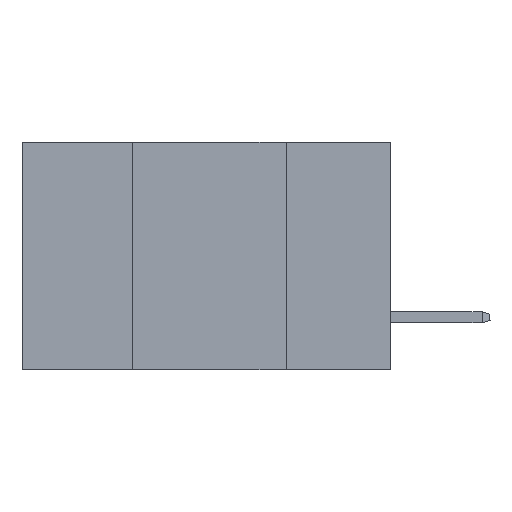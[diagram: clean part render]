
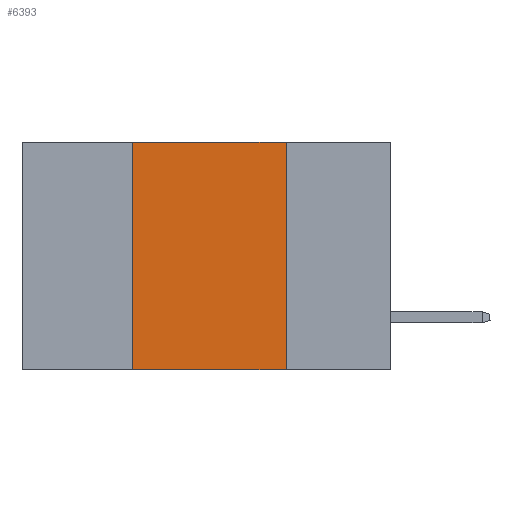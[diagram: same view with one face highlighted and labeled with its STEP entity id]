
A CAD part, left-side view. The second image highlights one B-rep face of the part: STEP entity #6393.
In plain terms, the highlighted planar face has unit normal (-1, 0, 0).
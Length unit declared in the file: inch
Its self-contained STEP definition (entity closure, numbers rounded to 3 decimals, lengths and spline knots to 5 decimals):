
#67 = EDGE_CURVE ( 'NONE', #12424, #2260, #8202, .T. ) ;
#159 = CARTESIAN_POINT ( 'NONE',  ( 0., 0.42, -0.37 ) ) ;
#267 = VECTOR ( 'NONE', #10061, 39.37008 ) ;
#717 = ORIENTED_EDGE ( 'NONE', *, *, #6623, .T. ) ;
#1902 = DIRECTION ( 'NONE',  ( 0., 0., 1. ) ) ;
#2260 = VERTEX_POINT ( 'NONE', #13333 ) ;
#2821 = LINE ( 'NONE', #7608, #267 ) ;
#3528 = ORIENTED_EDGE ( 'NONE', *, *, #14683, .F. ) ;
#3998 = VECTOR ( 'NONE', #12042, 39.37008 ) ;
#4241 = PLANE ( 'NONE',  #13665 ) ;
#4263 = ORIENTED_EDGE ( 'NONE', *, *, #11151, .F. ) ;
#4367 = ORIENTED_EDGE ( 'NONE', *, *, #67, .F. ) ;
#5123 = VERTEX_POINT ( 'NONE', #7650 ) ;
#6393 = ADVANCED_FACE ( 'NONE', ( #9859 ), #4241, .F. ) ;
#6436 = VERTEX_POINT ( 'NONE', #12186 ) ;
#6503 = CARTESIAN_POINT ( 'NONE',  ( 0., 0.42, 0. ) ) ;
#6623 = EDGE_CURVE ( 'NONE', #12424, #5123, #2821, .T. ) ;
#7331 = CARTESIAN_POINT ( 'NONE',  ( 0., 0.17, 0. ) ) ;
#7527 = DIRECTION ( 'NONE',  ( 1., 0., 0. ) ) ;
#7608 = CARTESIAN_POINT ( 'NONE',  ( 0., 0.6, -0.37 ) ) ;
#7650 = CARTESIAN_POINT ( 'NONE',  ( 0., 0.17, -0.37 ) ) ;
#8202 = LINE ( 'NONE', #6503, #9123 ) ;
#8470 = DIRECTION ( 'NONE',  ( 0., 0., -1. ) ) ;
#9123 = VECTOR ( 'NONE', #1902, 39.37008 ) ;
#9859 = FACE_OUTER_BOUND ( 'NONE', #10830, .T. ) ;
#10061 = DIRECTION ( 'NONE',  ( 0., -1., 0. ) ) ;
#10660 = CARTESIAN_POINT ( 'NONE',  ( 0., 0.6, 0. ) ) ;
#10789 = LINE ( 'NONE', #7331, #14103 ) ;
#10830 = EDGE_LOOP ( 'NONE', ( #4263, #3528, #4367, #717 ) ) ;
#10972 = DIRECTION ( 'NONE',  ( 0., 0., -1. ) ) ;
#11151 = EDGE_CURVE ( 'NONE', #6436, #5123, #10789, .T. ) ;
#12042 = DIRECTION ( 'NONE',  ( 0., -1., 0. ) ) ;
#12186 = CARTESIAN_POINT ( 'NONE',  ( 0., 0.17, 0. ) ) ;
#12424 = VERTEX_POINT ( 'NONE', #159 ) ;
#13333 = CARTESIAN_POINT ( 'NONE',  ( 0., 0.42, 0. ) ) ;
#13541 = CARTESIAN_POINT ( 'NONE',  ( 0., 0.6, 0. ) ) ;
#13665 = AXIS2_PLACEMENT_3D ( 'NONE', #13541, #7527, #10972 ) ;
#13997 = LINE ( 'NONE', #10660, #3998 ) ;
#14103 = VECTOR ( 'NONE', #8470, 39.37008 ) ;
#14683 = EDGE_CURVE ( 'NONE', #2260, #6436, #13997, .T. ) ;
